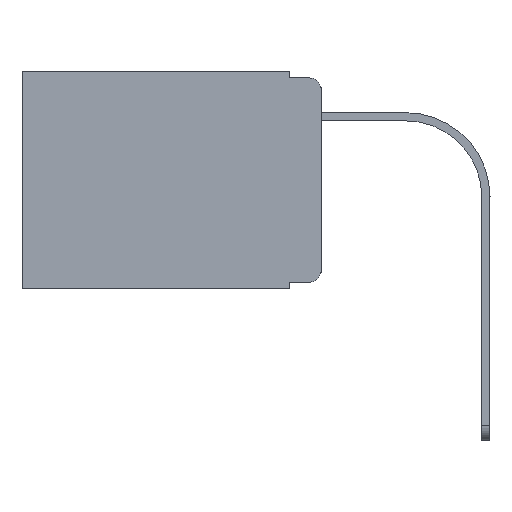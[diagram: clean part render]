
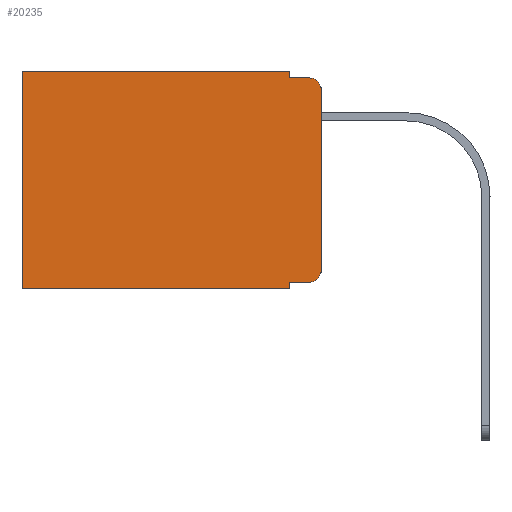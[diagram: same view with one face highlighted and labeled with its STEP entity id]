
A CAD part, left-side view. The second image highlights one B-rep face of the part: STEP entity #20235.
In plain terms, the highlighted planar face has unit normal (-1, 0, 0).
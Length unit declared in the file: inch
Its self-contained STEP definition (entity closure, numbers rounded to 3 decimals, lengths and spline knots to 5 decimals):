
#175 = CARTESIAN_POINT ( 'NONE',  ( 0.298, 0., -0.343 ) ) ;
#292 = CARTESIAN_POINT ( 'NONE',  ( 0.298, 0., 0. ) ) ;
#314 = VECTOR ( 'NONE', #12169, 39.37008 ) ;
#692 = DIRECTION ( 'NONE',  ( 0., 0., -1. ) ) ;
#785 = CARTESIAN_POINT ( 'NONE',  ( 0.298, 0., 0. ) ) ;
#1073 = VERTEX_POINT ( 'NONE', #11100 ) ;
#1391 = LINE ( 'NONE', #20307, #17753 ) ;
#1439 = LINE ( 'NONE', #2792, #15701 ) ;
#2792 = CARTESIAN_POINT ( 'NONE',  ( 0.298, 0., 0. ) ) ;
#2794 = EDGE_CURVE ( 'NONE', #6123, #6502, #19644, .T. ) ;
#3702 = LINE ( 'NONE', #5656, #8168 ) ;
#4448 = ORIENTED_EDGE ( 'NONE', *, *, #15425, .F. ) ;
#4457 = AXIS2_PLACEMENT_3D ( 'NONE', #6529, #17298, #11180 ) ;
#4528 = VERTEX_POINT ( 'NONE', #5070 ) ;
#4620 = CARTESIAN_POINT ( 'NONE',  ( 0.298, 0.02, -0.01 ) ) ;
#5023 = FACE_OUTER_BOUND ( 'NONE', #11844, .T. ) ;
#5069 = EDGE_CURVE ( 'NONE', #4528, #18614, #3702, .T. ) ;
#5070 = CARTESIAN_POINT ( 'NONE',  ( 0.298, 0.473, 0. ) ) ;
#5112 = CARTESIAN_POINT ( 'NONE',  ( 0.298, 0., -0.313 ) ) ;
#5159 = CARTESIAN_POINT ( 'NONE',  ( 0.298, 0., -0.03 ) ) ;
#5231 = LINE ( 'NONE', #785, #18070 ) ;
#5232 = DIRECTION ( 'NONE',  ( 1., 0., 0. ) ) ;
#5484 = EDGE_CURVE ( 'NONE', #14380, #1073, #18163, .T. ) ;
#5656 = CARTESIAN_POINT ( 'NONE',  ( 0.298, 0.473, 0. ) ) ;
#5687 = CARTESIAN_POINT ( 'NONE',  ( 0.298, 0.051, -0.01 ) ) ;
#5848 = DIRECTION ( 'NONE',  ( 0., 0., -1. ) ) ;
#6123 = VERTEX_POINT ( 'NONE', #5159 ) ;
#6393 = EDGE_CURVE ( 'NONE', #11867, #17160, #10821, .T. ) ;
#6470 = DIRECTION ( 'NONE',  ( 0., 1., 0. ) ) ;
#6502 = VERTEX_POINT ( 'NONE', #4620 ) ;
#6529 = CARTESIAN_POINT ( 'NONE',  ( 0.298, 0.02, -0.03 ) ) ;
#6669 = PLANE ( 'NONE',  #16831 ) ;
#7687 = DIRECTION ( 'NONE',  ( 0., 0., -1. ) ) ;
#8168 = VECTOR ( 'NONE', #18092, 39.37008 ) ;
#8338 = CARTESIAN_POINT ( 'NONE',  ( 0.298, 0.051, -0.333 ) ) ;
#8471 = EDGE_CURVE ( 'NONE', #1073, #10071, #17602, .T. ) ;
#8674 = AXIS2_PLACEMENT_3D ( 'NONE', #8953, #10402, #5848 ) ;
#8953 = CARTESIAN_POINT ( 'NONE',  ( 0.298, 0.02, -0.313 ) ) ;
#9088 = DIRECTION ( 'NONE',  ( 0., 0., -1. ) ) ;
#9203 = LINE ( 'NONE', #5687, #11056 ) ;
#9276 = ORIENTED_EDGE ( 'NONE', *, *, #12413, .F. ) ;
#9401 = CARTESIAN_POINT ( 'NONE',  ( 0.298, 0.473, -0.343 ) ) ;
#9538 = ORIENTED_EDGE ( 'NONE', *, *, #8471, .T. ) ;
#10071 = VERTEX_POINT ( 'NONE', #5112 ) ;
#10284 = CARTESIAN_POINT ( 'NONE',  ( 0.298, 0.051, -0.333 ) ) ;
#10345 = DIRECTION ( 'NONE',  ( 0., -1., 0. ) ) ;
#10402 = DIRECTION ( 'NONE',  ( -1., 0., 0. ) ) ;
#10607 = ORIENTED_EDGE ( 'NONE', *, *, #17571, .F. ) ;
#10821 = LINE ( 'NONE', #16854, #314 ) ;
#11056 = VECTOR ( 'NONE', #10345, 39.37008 ) ;
#11100 = CARTESIAN_POINT ( 'NONE',  ( 0.298, 0.02, -0.333 ) ) ;
#11126 = EDGE_CURVE ( 'NONE', #15981, #18614, #15891, .T. ) ;
#11180 = DIRECTION ( 'NONE',  ( 0., 0., -1. ) ) ;
#11529 = DIRECTION ( 'NONE',  ( 0., 1., 0. ) ) ;
#11844 = EDGE_LOOP ( 'NONE', ( #4448, #14347, #9276, #19963, #19007, #15736, #15558, #10607, #12416, #9538 ) ) ;
#11867 = VERTEX_POINT ( 'NONE', #15639 ) ;
#12169 = DIRECTION ( 'NONE',  ( 0., 0., -1. ) ) ;
#12413 = EDGE_CURVE ( 'NONE', #17160, #6502, #9203, .T. ) ;
#12416 = ORIENTED_EDGE ( 'NONE', *, *, #5484, .T. ) ;
#13329 = VECTOR ( 'NONE', #6470, 39.37008 ) ;
#13724 = CARTESIAN_POINT ( 'NONE',  ( 0.298, 0.051, -0.01 ) ) ;
#14347 = ORIENTED_EDGE ( 'NONE', *, *, #2794, .T. ) ;
#14380 = VERTEX_POINT ( 'NONE', #8338 ) ;
#14851 = DIRECTION ( 'NONE',  ( 0., -1., 0. ) ) ;
#15425 = EDGE_CURVE ( 'NONE', #6123, #10071, #1439, .T. ) ;
#15558 = ORIENTED_EDGE ( 'NONE', *, *, #11126, .F. ) ;
#15639 = CARTESIAN_POINT ( 'NONE',  ( 0.298, 0.051, 0. ) ) ;
#15701 = VECTOR ( 'NONE', #9088, 39.37008 ) ;
#15736 = ORIENTED_EDGE ( 'NONE', *, *, #5069, .T. ) ;
#15891 = LINE ( 'NONE', #175, #13329 ) ;
#15981 = VERTEX_POINT ( 'NONE', #17452 ) ;
#16786 = VECTOR ( 'NONE', #14851, 39.37008 ) ;
#16831 = AXIS2_PLACEMENT_3D ( 'NONE', #292, #5232, #692 ) ;
#16854 = CARTESIAN_POINT ( 'NONE',  ( 0.298, 0.051, 0. ) ) ;
#17160 = VERTEX_POINT ( 'NONE', #13724 ) ;
#17298 = DIRECTION ( 'NONE',  ( -1., 0., 0. ) ) ;
#17376 = EDGE_CURVE ( 'NONE', #11867, #4528, #5231, .T. ) ;
#17452 = CARTESIAN_POINT ( 'NONE',  ( 0.298, 0.051, -0.343 ) ) ;
#17571 = EDGE_CURVE ( 'NONE', #14380, #15981, #1391, .T. ) ;
#17602 = CIRCLE ( 'NONE', #8674, 0.02 ) ;
#17753 = VECTOR ( 'NONE', #7687, 39.37008 ) ;
#18070 = VECTOR ( 'NONE', #11529, 39.37008 ) ;
#18092 = DIRECTION ( 'NONE',  ( 0., 0., -1. ) ) ;
#18163 = LINE ( 'NONE', #10284, #16786 ) ;
#18614 = VERTEX_POINT ( 'NONE', #9401 ) ;
#19007 = ORIENTED_EDGE ( 'NONE', *, *, #17376, .T. ) ;
#19644 = CIRCLE ( 'NONE', #4457, 0.02 ) ;
#19963 = ORIENTED_EDGE ( 'NONE', *, *, #6393, .F. ) ;
#20235 = ADVANCED_FACE ( 'NONE', ( #5023 ), #6669, .F. ) ;
#20307 = CARTESIAN_POINT ( 'NONE',  ( 0.298, 0.051, 0. ) ) ;
